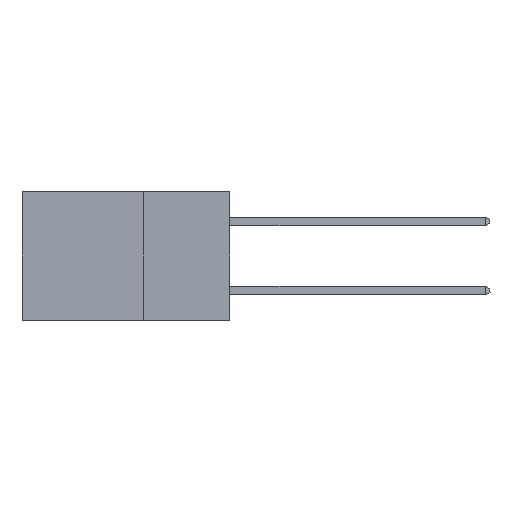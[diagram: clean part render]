
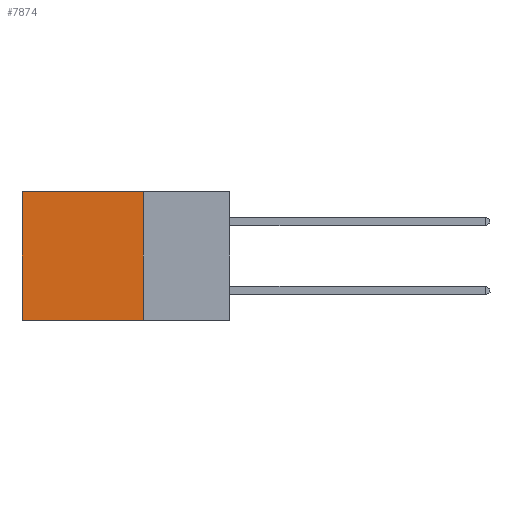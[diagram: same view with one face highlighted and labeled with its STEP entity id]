
A CAD part, left-side view. The second image highlights one B-rep face of the part: STEP entity #7874.
In plain terms, the highlighted planar face has unit normal (-1, 0, 0).
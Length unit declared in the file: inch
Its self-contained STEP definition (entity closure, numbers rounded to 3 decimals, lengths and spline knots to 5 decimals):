
#61 = EDGE_CURVE ( 'NONE', #16789, #282, #4560, .T. ) ;
#282 = VERTEX_POINT ( 'NONE', #2701 ) ;
#1212 = VECTOR ( 'NONE', #2782, 39.37008 ) ;
#2701 = CARTESIAN_POINT ( 'NONE',  ( 0.298, 0.6, -0.37 ) ) ;
#2782 = DIRECTION ( 'NONE',  ( 0., 1., 0. ) ) ;
#3495 = VERTEX_POINT ( 'NONE', #17336 ) ;
#4040 = DIRECTION ( 'NONE',  ( 1., 0., 0. ) ) ;
#4457 = EDGE_CURVE ( 'NONE', #3495, #12100, #11116, .T. ) ;
#4560 = LINE ( 'NONE', #7021, #7284 ) ;
#5792 = EDGE_CURVE ( 'NONE', #3495, #16789, #9192, .T. ) ;
#6478 = LINE ( 'NONE', #10838, #1212 ) ;
#6637 = CARTESIAN_POINT ( 'NONE',  ( 0.298, 0.25, 0. ) ) ;
#6816 = DIRECTION ( 'NONE',  ( 0., 0., -1. ) ) ;
#7021 = CARTESIAN_POINT ( 'NONE',  ( 0.298, 0.6, 0. ) ) ;
#7284 = VECTOR ( 'NONE', #14821, 39.37008 ) ;
#7874 = ADVANCED_FACE ( 'NONE', ( #10533 ), #17328, .F. ) ;
#8998 = ORIENTED_EDGE ( 'NONE', *, *, #4457, .F. ) ;
#9192 = LINE ( 'NONE', #16378, #10650 ) ;
#9379 = ORIENTED_EDGE ( 'NONE', *, *, #61, .T. ) ;
#9832 = VECTOR ( 'NONE', #10749, 39.37008 ) ;
#9918 = EDGE_CURVE ( 'NONE', #12100, #282, #6478, .T. ) ;
#10533 = FACE_OUTER_BOUND ( 'NONE', #17141, .T. ) ;
#10650 = VECTOR ( 'NONE', #13599, 39.37008 ) ;
#10749 = DIRECTION ( 'NONE',  ( 0., 0., -1. ) ) ;
#10838 = CARTESIAN_POINT ( 'NONE',  ( 0.298, 0.25, -0.37 ) ) ;
#11116 = LINE ( 'NONE', #17350, #9832 ) ;
#11285 = AXIS2_PLACEMENT_3D ( 'NONE', #6637, #4040, #6816 ) ;
#11569 = CARTESIAN_POINT ( 'NONE',  ( 0.298, 0.25, -0.37 ) ) ;
#12100 = VERTEX_POINT ( 'NONE', #11569 ) ;
#12920 = ORIENTED_EDGE ( 'NONE', *, *, #5792, .T. ) ;
#13599 = DIRECTION ( 'NONE',  ( 0., 1., 0. ) ) ;
#14821 = DIRECTION ( 'NONE',  ( 0., 0., -1. ) ) ;
#16378 = CARTESIAN_POINT ( 'NONE',  ( 0.298, 0.25, 0. ) ) ;
#16540 = CARTESIAN_POINT ( 'NONE',  ( 0.298, 0.6, 0. ) ) ;
#16789 = VERTEX_POINT ( 'NONE', #16540 ) ;
#17141 = EDGE_LOOP ( 'NONE', ( #9379, #17174, #8998, #12920 ) ) ;
#17174 = ORIENTED_EDGE ( 'NONE', *, *, #9918, .F. ) ;
#17328 = PLANE ( 'NONE',  #11285 ) ;
#17336 = CARTESIAN_POINT ( 'NONE',  ( 0.298, 0.25, 0. ) ) ;
#17350 = CARTESIAN_POINT ( 'NONE',  ( 0.298, 0.25, 0. ) ) ;
